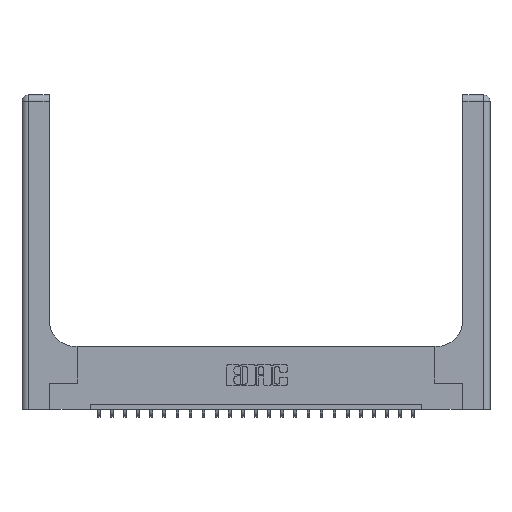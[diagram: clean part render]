
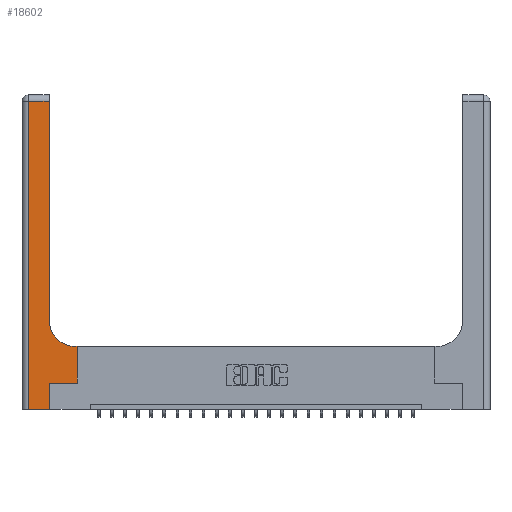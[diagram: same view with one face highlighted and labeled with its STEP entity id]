
A CAD part, top view. The second image highlights one B-rep face of the part: STEP entity #18602.
In plain terms, the highlighted planar face has unit normal (0, 0, 1).
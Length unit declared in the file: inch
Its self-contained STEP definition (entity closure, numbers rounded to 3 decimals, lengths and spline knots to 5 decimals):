
#408 = CARTESIAN_POINT ( 'NONE',  ( 0.265, 0.25, 0.37 ) ) ;
#640 = CARTESIAN_POINT ( 'NONE',  ( 0.51, 0.85, 0.37 ) ) ;
#717 = VERTEX_POINT ( 'NONE', #7558 ) ;
#760 = ORIENTED_EDGE ( 'NONE', *, *, #13896, .T. ) ;
#1103 = CARTESIAN_POINT ( 'NONE',  ( 0.06, 2.94, 0.37 ) ) ;
#1310 = FACE_OUTER_BOUND ( 'NONE', #15851, .T. ) ;
#1397 = CARTESIAN_POINT ( 'NONE',  ( 0.528, 0.6, 0.37 ) ) ;
#1681 = DIRECTION ( 'NONE',  ( 0., -1., 0. ) ) ;
#1682 = LINE ( 'NONE', #7961, #20099 ) ;
#2432 = DIRECTION ( 'NONE',  ( 1., 0., 0. ) ) ;
#2706 = ORIENTED_EDGE ( 'NONE', *, *, #17203, .T. ) ;
#2946 = EDGE_CURVE ( 'NONE', #3306, #717, #11828, .T. ) ;
#3260 = ORIENTED_EDGE ( 'NONE', *, *, #3995, .T. ) ;
#3306 = VERTEX_POINT ( 'NONE', #6975 ) ;
#3612 = VECTOR ( 'NONE', #1681, 39.37008 ) ;
#3628 = VERTEX_POINT ( 'NONE', #20260 ) ;
#3754 = AXIS2_PLACEMENT_3D ( 'NONE', #22893, #8788, #21214 ) ;
#3811 = CARTESIAN_POINT ( 'NONE',  ( 0.26, 3., 0.37 ) ) ;
#3995 = EDGE_CURVE ( 'NONE', #22562, #13790, #4184, .T. ) ;
#4184 = LINE ( 'NONE', #22996, #3612 ) ;
#4206 = DIRECTION ( 'NONE',  ( 1., 0., 0. ) ) ;
#4927 = VERTEX_POINT ( 'NONE', #1397 ) ;
#4964 = ORIENTED_EDGE ( 'NONE', *, *, #22232, .T. ) ;
#6720 = DIRECTION ( 'NONE',  ( -1., 0., 0. ) ) ;
#6749 = CARTESIAN_POINT ( 'NONE',  ( 0.265, 0., 0.37 ) ) ;
#6975 = CARTESIAN_POINT ( 'NONE',  ( 0.51, 0.6, 0.37 ) ) ;
#7371 = EDGE_CURVE ( 'NONE', #17098, #3628, #18103, .T. ) ;
#7558 = CARTESIAN_POINT ( 'NONE',  ( 0.26, 0.85, 0.37 ) ) ;
#7835 = VECTOR ( 'NONE', #14563, 39.37008 ) ;
#7961 = CARTESIAN_POINT ( 'NONE',  ( 0.528, 0.25, 0.37 ) ) ;
#8119 = VECTOR ( 'NONE', #20955, 39.37008 ) ;
#8192 = VECTOR ( 'NONE', #11396, 39.37008 ) ;
#8788 = DIRECTION ( 'NONE',  ( 0., 0., -1. ) ) ;
#8897 = VECTOR ( 'NONE', #6720, 39.37008 ) ;
#9048 = LINE ( 'NONE', #21367, #22643 ) ;
#9583 = CARTESIAN_POINT ( 'NONE',  ( 0.06, 0., 0.37 ) ) ;
#10853 = ORIENTED_EDGE ( 'NONE', *, *, #2946, .T. ) ;
#11396 = DIRECTION ( 'NONE',  ( -1., 0., 0. ) ) ;
#11828 = CIRCLE ( 'NONE', #19819, 0.25 ) ;
#12562 = DIRECTION ( 'NONE',  ( 1., 0., 0. ) ) ;
#12746 = EDGE_CURVE ( 'NONE', #12855, #17098, #22264, .T. ) ;
#12855 = VERTEX_POINT ( 'NONE', #21256 ) ;
#12984 = EDGE_CURVE ( 'NONE', #717, #19140, #21981, .T. ) ;
#13207 = DIRECTION ( 'NONE',  ( 0., 0., -1. ) ) ;
#13790 = VERTEX_POINT ( 'NONE', #9583 ) ;
#13818 = CARTESIAN_POINT ( 'NONE',  ( 0.26, 2.94, 0.37 ) ) ;
#13896 = EDGE_CURVE ( 'NONE', #4927, #3306, #17809, .T. ) ;
#14563 = DIRECTION ( 'NONE',  ( 0., 1., 0. ) ) ;
#15851 = EDGE_LOOP ( 'NONE', ( #16438, #2706, #3260, #22209, #18074, #18632, #4964, #760, #10853 ) ) ;
#16438 = ORIENTED_EDGE ( 'NONE', *, *, #12984, .T. ) ;
#16489 = EDGE_CURVE ( 'NONE', #13790, #12855, #9048, .T. ) ;
#17098 = VERTEX_POINT ( 'NONE', #408 ) ;
#17203 = EDGE_CURVE ( 'NONE', #19140, #22562, #17660, .T. ) ;
#17398 = CARTESIAN_POINT ( 'NONE',  ( 0.26, 0.6, 0.37 ) ) ;
#17553 = VECTOR ( 'NONE', #4206, 39.37008 ) ;
#17660 = LINE ( 'NONE', #21976, #8192 ) ;
#17809 = LINE ( 'NONE', #17398, #8897 ) ;
#18074 = ORIENTED_EDGE ( 'NONE', *, *, #12746, .T. ) ;
#18103 = LINE ( 'NONE', #20254, #17553 ) ;
#18602 = ADVANCED_FACE ( 'NONE', ( #1310 ), #19433, .F. ) ;
#18632 = ORIENTED_EDGE ( 'NONE', *, *, #7371, .T. ) ;
#19140 = VERTEX_POINT ( 'NONE', #13818 ) ;
#19433 = PLANE ( 'NONE',  #3754 ) ;
#19819 = AXIS2_PLACEMENT_3D ( 'NONE', #640, #13207, #2432 ) ;
#20099 = VECTOR ( 'NONE', #20446, 39.37008 ) ;
#20254 = CARTESIAN_POINT ( 'NONE',  ( 0.265, 0.25, 0.37 ) ) ;
#20260 = CARTESIAN_POINT ( 'NONE',  ( 0.528, 0.25, 0.37 ) ) ;
#20446 = DIRECTION ( 'NONE',  ( 0., 1., 0. ) ) ;
#20955 = DIRECTION ( 'NONE',  ( 0., 1., 0. ) ) ;
#21214 = DIRECTION ( 'NONE',  ( -1., 0., 0. ) ) ;
#21256 = CARTESIAN_POINT ( 'NONE',  ( 0.265, 0., 0.37 ) ) ;
#21367 = CARTESIAN_POINT ( 'NONE',  ( 0., 0., 0.37 ) ) ;
#21976 = CARTESIAN_POINT ( 'NONE',  ( 0., 2.94, 0.37 ) ) ;
#21981 = LINE ( 'NONE', #3811, #7835 ) ;
#22209 = ORIENTED_EDGE ( 'NONE', *, *, #16489, .T. ) ;
#22232 = EDGE_CURVE ( 'NONE', #3628, #4927, #1682, .T. ) ;
#22264 = LINE ( 'NONE', #6749, #8119 ) ;
#22562 = VERTEX_POINT ( 'NONE', #1103 ) ;
#22643 = VECTOR ( 'NONE', #12562, 39.37008 ) ;
#22893 = CARTESIAN_POINT ( 'NONE',  ( 0., 3., 0.37 ) ) ;
#22996 = CARTESIAN_POINT ( 'NONE',  ( 0.06, 3., 0.37 ) ) ;
